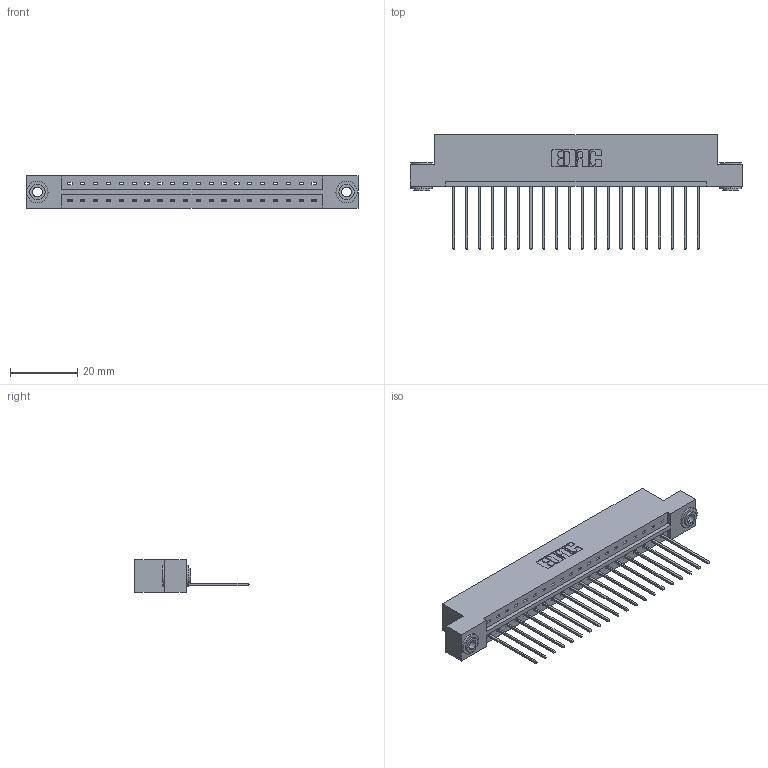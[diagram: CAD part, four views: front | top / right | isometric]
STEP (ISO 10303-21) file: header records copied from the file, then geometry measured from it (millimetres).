
FILE_DESCRIPTION (( 'STEP AP203' ), '1' );
FILE_NAME ('379-020-541-103.STEP', '2020-02-26T15:13:19', ( '' ), ( '' ), 'SwSTEP 2.0', 'SolidWorks 2016', '' );
FILE_SCHEMA (( 'CONFIG_CONTROL_DESIGN' ));
Length unit declared in the file: inch
Products named in the file (4): 345-292-001_345-293-141; 345-250-002_345-250-002-102; 379-020-541-103; 379 Part_Flush - .156 Dia - TH
Assembly tree (23 placements, depth 2):
  379-020-541-103
    379 Part_Flush - .156 Dia - TH
    345-292-001_345-293-141  x20
    345-250-002_345-250-002-102  x2
Bounding box: 98.42 x 33.96 x 9.53 mm (x, y, z)
Volume: 10164 mm3; surface area: 10929.7 mm2
Topology: 23 solids, 23 shells, 1312 faces, 3907 edges, 2574 vertices
Faces by surface type: plane 920, cylinder 384, cone 8
Entity records: 15740 total; most frequent: CARTESIAN_POINT 2697, ORIENTED_EDGE 2646, DIRECTION 2353, EDGE_CURVE 1323, VECTOR 1171, LINE 1171, VERTEX_POINT 878, AXIS2_PLACEMENT_3D 591
